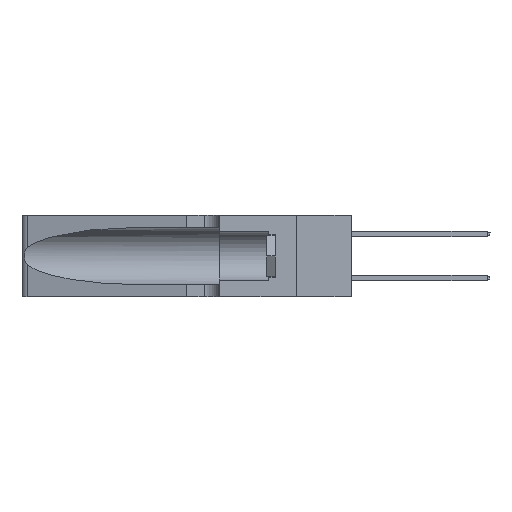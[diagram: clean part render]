
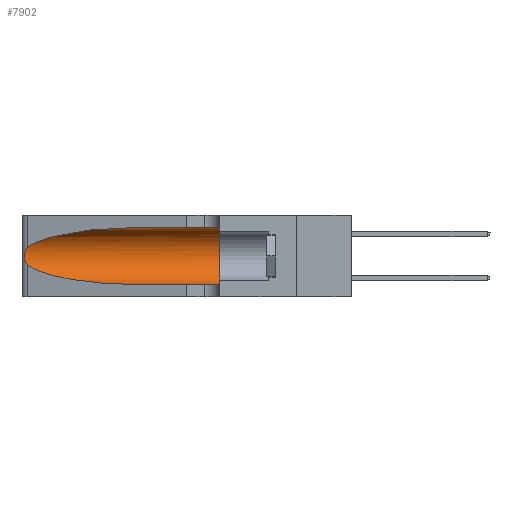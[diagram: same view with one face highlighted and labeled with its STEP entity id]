
A CAD part, left-side view. The second image highlights one B-rep face of the part: STEP entity #7902.
In plain terms, the highlighted cylindrical face has radius 3.308 mm (diameter 6.617 mm), a partial arc.
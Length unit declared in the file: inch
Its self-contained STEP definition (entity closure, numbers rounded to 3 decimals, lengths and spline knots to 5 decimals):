
#721 = CARTESIAN_POINT ( 'NONE',  ( 0.25487, 1.22718, 0.22369 ) ) ;
#877 = CARTESIAN_POINT ( 'NONE',  ( 0.25487, 1.22718, 0.14631 ) ) ;
#2118 = B_SPLINE_CURVE_WITH_KNOTS ( 'NONE', 3,
 ( #721, #22703, #4464, #29907, #8185, #33485, #11898, #37047, #15621, #40629, #19261, #44204, #22855, #877 ),
 .UNSPECIFIED., .F., .F.,
 ( 4, 2, 2, 2, 2, 2, 4 ),
 ( 0., 0.00027, 0.00053, 0.00107, 0.0016, 0.00187, 0.00214 ),
 .UNSPECIFIED. ) ;
#2222 = EDGE_CURVE ( 'NONE', #20727, #23641, #31010, .T. ) ;
#2493 = DIRECTION ( 'NONE',  ( 0., -1., 0. ) ) ;
#3435 = VERTEX_POINT ( 'NONE', #25874 ) ;
#3585 = DIRECTION ( 'NONE',  ( 0., 1., 0. ) ) ;
#4464 = CARTESIAN_POINT ( 'NONE',  ( 0.25639, 1.23184, 0.21858 ) ) ;
#5623 = LINE ( 'NONE', #46188, #23903 ) ;
#5649 = VERTEX_POINT ( 'NONE', #8680 ) ;
#6709 = CARTESIAN_POINT ( 'NONE',  ( 0.18966, 0.96281, 0.05475 ) ) ;
#7029 = ORIENTED_EDGE ( 'NONE', *, *, #12489, .T. ) ;
#7276 = ORIENTED_EDGE ( 'NONE', *, *, #2222, .T. ) ;
#7902 = ADVANCED_FACE ( 'NONE', ( #17906 ), #16768, .F. ) ;
#8185 = CARTESIAN_POINT ( 'NONE',  ( 0.25854, 1.2359, 0.20912 ) ) ;
#8680 = CARTESIAN_POINT ( 'NONE',  ( 0.1305, 0.72297, 0.05475 ) ) ;
#10231 = CARTESIAN_POINT ( 'NONE',  ( 0.25487, 1.22718, 0.22369 ) ) ;
#11814 = CIRCLE ( 'NONE', #39494, 0.13025 ) ;
#11898 = CARTESIAN_POINT ( 'NONE',  ( 0.26075, 1.23896, 0.19203 ) ) ;
#12008 = CARTESIAN_POINT ( 'NONE',  ( 0.1305, 0.35, 0.31525 ) ) ;
#12489 = EDGE_CURVE ( 'NONE', #3435, #5649, #14293, .T. ) ;
#14293 =( BOUNDED_CURVE ( )  B_SPLINE_CURVE ( 3, ( #42663, #24887, #6709, #32063 ),
 .UNSPECIFIED., .F., .F. ) 
 B_SPLINE_CURVE_WITH_KNOTS ( ( 4, 4 ),
 ( 3.44316, 4.71239 ),
 .UNSPECIFIED. ) 
 CURVE ( )  GEOMETRIC_REPRESENTATION_ITEM ( )  RATIONAL_B_SPLINE_CURVE ( ( 1., 0.87, 0.87, 1. ) ) 
 REPRESENTATION_ITEM ( '' )  );
#15120 = VECTOR ( 'NONE', #44838, 39.37008 ) ;
#15424 = EDGE_CURVE ( 'NONE', #20727, #27337, #5623, .T. ) ;
#15621 = CARTESIAN_POINT ( 'NONE',  ( 0.26017, 1.23833, 0.17102 ) ) ;
#16665 = VERTEX_POINT ( 'NONE', #39099 ) ;
#16768 = CYLINDRICAL_SURFACE ( 'NONE', #32877, 0.13025 ) ;
#17906 = FACE_OUTER_BOUND ( 'NONE', #42832, .T. ) ;
#19261 = CARTESIAN_POINT ( 'NONE',  ( 0.25789, 1.23486, 0.15765 ) ) ;
#19861 = CARTESIAN_POINT ( 'NONE',  ( 0.25487, 1.22718, 0.22369 ) ) ;
#20727 = VERTEX_POINT ( 'NONE', #25386 ) ;
#21502 = ORIENTED_EDGE ( 'NONE', *, *, #15424, .F. ) ;
#22703 = CARTESIAN_POINT ( 'NONE',  ( 0.25555, 1.22994, 0.2215 ) ) ;
#22855 = CARTESIAN_POINT ( 'NONE',  ( 0.25555, 1.22993, 0.14849 ) ) ;
#23571 = LINE ( 'NONE', #41263, #15120 ) ;
#23639 = ORIENTED_EDGE ( 'NONE', *, *, #29720, .F. ) ;
#23641 = VERTEX_POINT ( 'NONE', #10231 ) ;
#23649 = ORIENTED_EDGE ( 'NONE', *, *, #31337, .T. ) ;
#23903 = VECTOR ( 'NONE', #28415, 39.37008 ) ;
#24392 = DIRECTION ( 'NONE',  ( 0., 0., -1. ) ) ;
#24887 = CARTESIAN_POINT ( 'NONE',  ( 0.2373, 1.15595, 0.08982 ) ) ;
#25386 = CARTESIAN_POINT ( 'NONE',  ( 0.1305, 0.72297, 0.31525 ) ) ;
#25464 = CARTESIAN_POINT ( 'NONE',  ( 0.1305, 0.35, 0.185 ) ) ;
#25874 = CARTESIAN_POINT ( 'NONE',  ( 0.25487, 1.22718, 0.14631 ) ) ;
#27337 = VERTEX_POINT ( 'NONE', #12008 ) ;
#28415 = DIRECTION ( 'NONE',  ( 0., -1., 0. ) ) ;
#29034 = DIRECTION ( 'NONE',  ( 0., 0., 1. ) ) ;
#29720 = EDGE_CURVE ( 'NONE', #27337, #16665, #11814, .T. ) ;
#29907 = CARTESIAN_POINT ( 'NONE',  ( 0.25787, 1.23484, 0.2124 ) ) ;
#30492 = CARTESIAN_POINT ( 'NONE',  ( 0.2373, 1.15595, 0.28018 ) ) ;
#31010 =( BOUNDED_CURVE ( )  B_SPLINE_CURVE ( 3, ( #41219, #34077, #30492, #19861 ),
 .UNSPECIFIED., .F., .F. ) 
 B_SPLINE_CURVE_WITH_KNOTS ( ( 4, 4 ),
 ( 1.5708, 2.84003 ),
 .UNSPECIFIED. ) 
 CURVE ( )  GEOMETRIC_REPRESENTATION_ITEM ( )  RATIONAL_B_SPLINE_CURVE ( ( 1., 0.87, 0.87, 1. ) ) 
 REPRESENTATION_ITEM ( '' )  );
#31337 = EDGE_CURVE ( 'NONE', #5649, #16665, #23571, .T. ) ;
#32063 = CARTESIAN_POINT ( 'NONE',  ( 0.1305, 0.72297, 0.05475 ) ) ;
#32877 = AXIS2_PLACEMENT_3D ( 'NONE', #45737, #2493, #24392 ) ;
#33485 = CARTESIAN_POINT ( 'NONE',  ( 0.26018, 1.23835, 0.19895 ) ) ;
#34077 = CARTESIAN_POINT ( 'NONE',  ( 0.18966, 0.96281, 0.31525 ) ) ;
#37047 = CARTESIAN_POINT ( 'NONE',  ( 0.26075, 1.23896, 0.178 ) ) ;
#37625 = EDGE_CURVE ( 'NONE', #23641, #3435, #2118, .T. ) ;
#38226 = ORIENTED_EDGE ( 'NONE', *, *, #37625, .T. ) ;
#39099 = CARTESIAN_POINT ( 'NONE',  ( 0.1305, 0.35, 0.05475 ) ) ;
#39494 = AXIS2_PLACEMENT_3D ( 'NONE', #25464, #3585, #29034 ) ;
#40629 = CARTESIAN_POINT ( 'NONE',  ( 0.25856, 1.23593, 0.16098 ) ) ;
#41219 = CARTESIAN_POINT ( 'NONE',  ( 0.1305, 0.72297, 0.31525 ) ) ;
#41263 = CARTESIAN_POINT ( 'NONE',  ( 0.1305, 1.61858, 0.05475 ) ) ;
#42663 = CARTESIAN_POINT ( 'NONE',  ( 0.25487, 1.22718, 0.14631 ) ) ;
#42832 = EDGE_LOOP ( 'NONE', ( #7276, #38226, #7029, #23649, #23639, #21502 ) ) ;
#44204 = CARTESIAN_POINT ( 'NONE',  ( 0.25639, 1.23186, 0.15144 ) ) ;
#44838 = DIRECTION ( 'NONE',  ( 0., -1., 0. ) ) ;
#45737 = CARTESIAN_POINT ( 'NONE',  ( 0.1305, 1.61858, 0.185 ) ) ;
#46188 = CARTESIAN_POINT ( 'NONE',  ( 0.1305, 1.61858, 0.31525 ) ) ;
